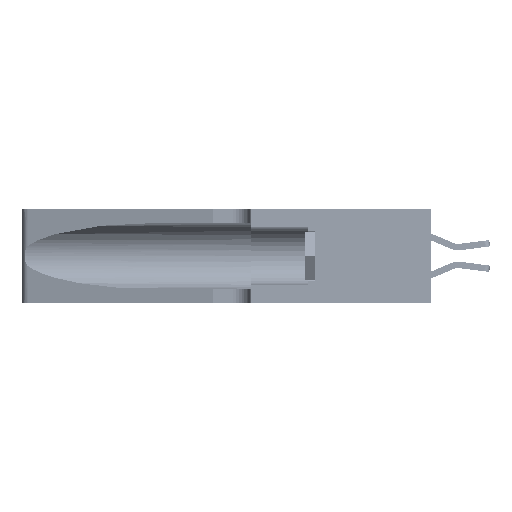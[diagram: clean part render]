
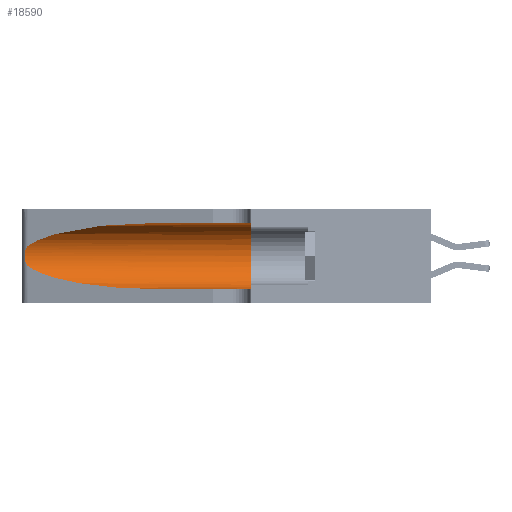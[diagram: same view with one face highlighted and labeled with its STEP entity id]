
A CAD part, left-side view. The second image highlights one B-rep face of the part: STEP entity #18590.
In plain terms, the highlighted cylindrical face has radius 3.308 mm (diameter 6.617 mm), a partial arc.
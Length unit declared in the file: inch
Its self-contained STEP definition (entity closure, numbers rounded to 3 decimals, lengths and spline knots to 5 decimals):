
#2077 = CARTESIAN_POINT ( 'NONE',  ( 0.2373, 1.15595, 0.08982 ) ) ;
#3237 = DIRECTION ( 'NONE',  ( 0., 0., 1. ) ) ;
#5115 = CARTESIAN_POINT ( 'NONE',  ( 0.25856, 1.23593, 0.16098 ) ) ;
#6887 = VECTOR ( 'NONE', #21256, 39.37008 ) ;
#7932 = DIRECTION ( 'NONE',  ( 0., -1., 0. ) ) ;
#8537 = CARTESIAN_POINT ( 'NONE',  ( 0.25854, 1.2359, 0.20912 ) ) ;
#8700 = CARTESIAN_POINT ( 'NONE',  ( 0.26075, 1.23896, 0.19203 ) ) ;
#9734 = CARTESIAN_POINT ( 'NONE',  ( 0.25487, 1.22718, 0.14631 ) ) ;
#10410 = CARTESIAN_POINT ( 'NONE',  ( 0.1305, 0.72297, 0.31525 ) ) ;
#10569 = CARTESIAN_POINT ( 'NONE',  ( 0.1305, 0.35, 0.185 ) ) ;
#11061 = DIRECTION ( 'NONE',  ( 0., 1., 0. ) ) ;
#11549 = CARTESIAN_POINT ( 'NONE',  ( 0.1305, 1.61858, 0.05475 ) ) ;
#12502 = CARTESIAN_POINT ( 'NONE',  ( 0.25639, 1.23186, 0.15144 ) ) ;
#12726 = CARTESIAN_POINT ( 'NONE',  ( 0.18966, 0.96281, 0.31525 ) ) ;
#14825 = ORIENTED_EDGE ( 'NONE', *, *, #24228, .T. ) ;
#15749 = DIRECTION ( 'NONE',  ( 0., -1., 0. ) ) ;
#17127 = EDGE_CURVE ( 'NONE', #42357, #37673, #21724, .T. ) ;
#17198 = AXIS2_PLACEMENT_3D ( 'NONE', #19226, #15749, #38356 ) ;
#17626 = CARTESIAN_POINT ( 'NONE',  ( 0.1305, 1.61858, 0.31525 ) ) ;
#18590 = ADVANCED_FACE ( 'NONE', ( #31472 ), #25066, .F. ) ;
#18600 = VERTEX_POINT ( 'NONE', #34731 ) ;
#19215 = AXIS2_PLACEMENT_3D ( 'NONE', #10569, #11061, #3237 ) ;
#19226 = CARTESIAN_POINT ( 'NONE',  ( 0.1305, 1.61858, 0.185 ) ) ;
#19776 = CARTESIAN_POINT ( 'NONE',  ( 0.26018, 1.23835, 0.19895 ) ) ;
#20111 = CARTESIAN_POINT ( 'NONE',  ( 0.25487, 1.22718, 0.22369 ) ) ;
#20178 = EDGE_CURVE ( 'NONE', #24523, #37673, #32086, .T. ) ;
#21256 = DIRECTION ( 'NONE',  ( 0., -1., 0. ) ) ;
#21724 = CIRCLE ( 'NONE', #19215, 0.13025 ) ;
#22419 = EDGE_CURVE ( 'NONE', #43464, #24523, #27983, .T. ) ;
#22727 = ORIENTED_EDGE ( 'NONE', *, *, #39608, .T. ) ;
#23887 = VECTOR ( 'NONE', #7932, 39.37008 ) ;
#24228 = EDGE_CURVE ( 'NONE', #43865, #18600, #45407, .T. ) ;
#24232 = CARTESIAN_POINT ( 'NONE',  ( 0.1305, 0.72297, 0.05475 ) ) ;
#24523 = VERTEX_POINT ( 'NONE', #34147 ) ;
#25066 = CYLINDRICAL_SURFACE ( 'NONE', #17198, 0.13025 ) ;
#26936 = ORIENTED_EDGE ( 'NONE', *, *, #22419, .T. ) ;
#26958 = ORIENTED_EDGE ( 'NONE', *, *, #17127, .F. ) ;
#27041 = CARTESIAN_POINT ( 'NONE',  ( 0.25487, 1.22718, 0.14631 ) ) ;
#27287 = EDGE_CURVE ( 'NONE', #43865, #42357, #40411, .T. ) ;
#27436 = CARTESIAN_POINT ( 'NONE',  ( 0.25487, 1.22718, 0.14631 ) ) ;
#27763 = CARTESIAN_POINT ( 'NONE',  ( 0.25639, 1.23184, 0.21858 ) ) ;
#27983 =( BOUNDED_CURVE ( )  B_SPLINE_CURVE ( 3, ( #9734, #2077, #28297, #24232 ),
 .UNSPECIFIED., .F., .T. ) 
 B_SPLINE_CURVE_WITH_KNOTS ( ( 4, 4 ),
 ( 3.44316, 4.71239 ),
 .UNSPECIFIED. ) 
 CURVE ( )  GEOMETRIC_REPRESENTATION_ITEM ( )  RATIONAL_B_SPLINE_CURVE ( ( 1., 0.87, 0.87, 1. ) ) 
 REPRESENTATION_ITEM ( '' )  );
#28297 = CARTESIAN_POINT ( 'NONE',  ( 0.18966, 0.96281, 0.05475 ) ) ;
#28371 = EDGE_LOOP ( 'NONE', ( #14825, #22727, #26936, #29926, #26958, #44961 ) ) ;
#29926 = ORIENTED_EDGE ( 'NONE', *, *, #20178, .T. ) ;
#31053 = CARTESIAN_POINT ( 'NONE',  ( 0.25555, 1.22994, 0.2215 ) ) ;
#31472 = FACE_OUTER_BOUND ( 'NONE', #28371, .T. ) ;
#32063 = CARTESIAN_POINT ( 'NONE',  ( 0.1305, 0.72297, 0.31525 ) ) ;
#32086 = LINE ( 'NONE', #11549, #23887 ) ;
#34147 = CARTESIAN_POINT ( 'NONE',  ( 0.1305, 0.72297, 0.05475 ) ) ;
#34731 = CARTESIAN_POINT ( 'NONE',  ( 0.25487, 1.22718, 0.22369 ) ) ;
#34955 = CARTESIAN_POINT ( 'NONE',  ( 0.25555, 1.22993, 0.14849 ) ) ;
#36167 = CARTESIAN_POINT ( 'NONE',  ( 0.2373, 1.15595, 0.28018 ) ) ;
#37288 = B_SPLINE_CURVE_WITH_KNOTS ( 'NONE', 3,
 ( #20111, #31053, #27763, #39080, #8537, #19776, #8700, #46346, #38751, #5115, #42872, #12502, #34955, #27436 ),
 .UNSPECIFIED., .F., .F.,
 ( 4, 2, 2, 2, 2, 2, 4 ),
 ( 0., 0.00027, 0.00053, 0.00107, 0.0016, 0.00187, 0.00214 ),
 .UNSPECIFIED. ) ;
#37673 = VERTEX_POINT ( 'NONE', #39236 ) ;
#38356 = DIRECTION ( 'NONE',  ( 0., 0., -1. ) ) ;
#38751 = CARTESIAN_POINT ( 'NONE',  ( 0.26017, 1.23833, 0.17102 ) ) ;
#38787 = CARTESIAN_POINT ( 'NONE',  ( 0.1305, 0.35, 0.31525 ) ) ;
#39080 = CARTESIAN_POINT ( 'NONE',  ( 0.25787, 1.23484, 0.2124 ) ) ;
#39236 = CARTESIAN_POINT ( 'NONE',  ( 0.1305, 0.35, 0.05475 ) ) ;
#39608 = EDGE_CURVE ( 'NONE', #18600, #43464, #37288, .T. ) ;
#40411 = LINE ( 'NONE', #17626, #6887 ) ;
#42357 = VERTEX_POINT ( 'NONE', #38787 ) ;
#42872 = CARTESIAN_POINT ( 'NONE',  ( 0.25789, 1.23486, 0.15765 ) ) ;
#43464 = VERTEX_POINT ( 'NONE', #27041 ) ;
#43865 = VERTEX_POINT ( 'NONE', #10410 ) ;
#44058 = CARTESIAN_POINT ( 'NONE',  ( 0.25487, 1.22718, 0.22369 ) ) ;
#44961 = ORIENTED_EDGE ( 'NONE', *, *, #27287, .F. ) ;
#45407 =( BOUNDED_CURVE ( )  B_SPLINE_CURVE ( 3, ( #32063, #12726, #36167, #44058 ),
 .UNSPECIFIED., .F., .F. ) 
 B_SPLINE_CURVE_WITH_KNOTS ( ( 4, 4 ),
 ( 1.5708, 2.84003 ),
 .UNSPECIFIED. ) 
 CURVE ( )  GEOMETRIC_REPRESENTATION_ITEM ( )  RATIONAL_B_SPLINE_CURVE ( ( 1., 0.87, 0.87, 1. ) ) 
 REPRESENTATION_ITEM ( '' )  );
#46346 = CARTESIAN_POINT ( 'NONE',  ( 0.26075, 1.23896, 0.178 ) ) ;
